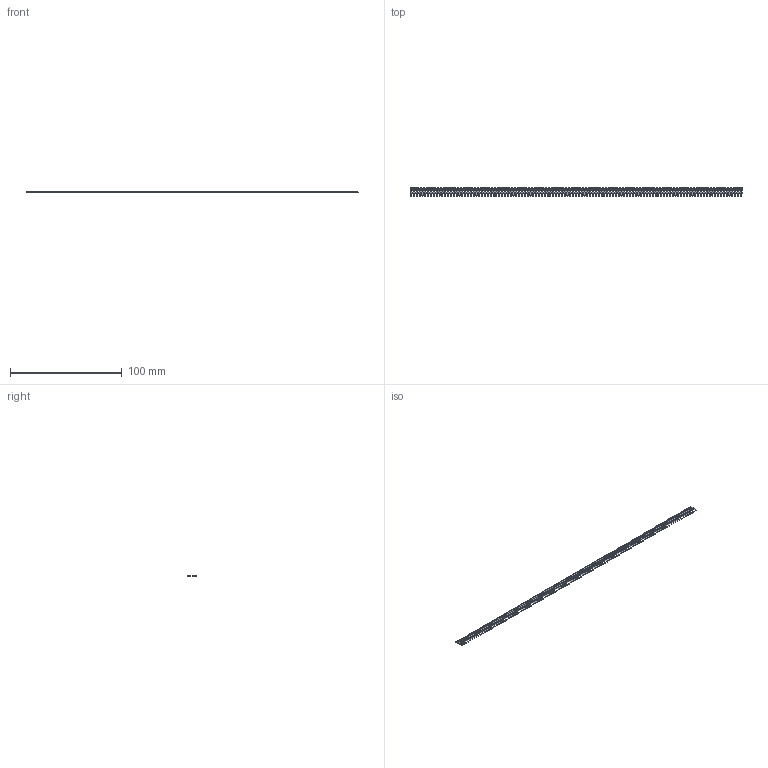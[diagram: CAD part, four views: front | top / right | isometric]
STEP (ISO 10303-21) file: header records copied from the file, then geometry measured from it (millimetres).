
FILE_DESCRIPTION (( 'STEP AP203' ), '1' );
FILE_NAME ('103-117-253-100.STEP', '2020-04-16T17:35:17', ( '' ), ( '' ), 'SwSTEP 2.0', 'SolidWorks 2016', '' );
FILE_SCHEMA (( 'CONFIG_CONTROL_DESIGN' ));
Length unit declared in the file: inch
Products named in the file (2): 100-290-001_100-290-253; 103-117-253-100
Assembly tree (117 placements, depth 2):
  103-117-253-100
    100-290-001_100-290-253  x117
Bounding box: 296.67 x 7.62 x 0.51 mm (x, y, z)
Volume: 645.6 mm3; surface area: 4025.6 mm2
Topology: 117 solids, 117 shells, 2340 faces, 6318 edges, 4212 vertices
Faces by surface type: plane 2223, cylinder 117
Entity records: 4532 total; most frequent: DIRECTION 336, DATE_AND_TIME 244, CALENDAR_DATE 244, LOCAL_TIME 244, COORDINATED_UNIVERSAL_TIME_OFFSET 244, CARTESIAN_POINT 230, AXIS2_PLACEMENT_3D 142, PERSON_AND_ORGANIZATION 133
